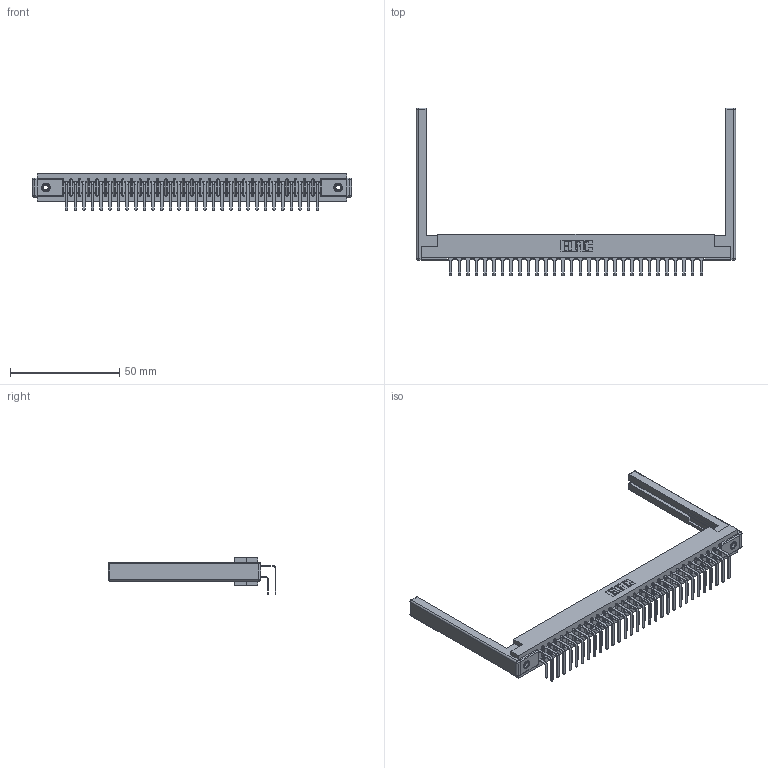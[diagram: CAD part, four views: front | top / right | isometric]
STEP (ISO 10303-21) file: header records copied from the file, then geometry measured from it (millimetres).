
FILE_DESCRIPTION (( 'STEP AP203' ), '1' );
FILE_NAME ('307-030-458-168.STEP', '2020-09-28T11:19:01', ( '' ), ( '' ), 'SwSTEP 2.0', 'SolidWorks 2020', '' );
FILE_SCHEMA (( 'CONFIG_CONTROL_DESIGN' ));
Length unit declared in the file: inch
Products named in the file (6): 307-030-458-168; 307 Part_.156 Dia Mounting Holes; 307-290-001_558 - 2 (Single); 345-250-001_345-250-001-102; 307-220-068; 307-290-001_558 559 - 1 (Single)
Assembly tree (65 placements, depth 2):
  307-030-458-168
    307 Part_.156 Dia Mounting Holes
    307-290-001_558 559 - 1 (Single)  x30
    307-290-001_558 - 2 (Single)  x30
    307-220-068  x2
    345-250-001_345-250-001-102  x2
Bounding box: 146.3 x 76.92 x 16.8 mm (x, y, z)
Volume: 20119.3 mm3; surface area: 24546.5 mm2
Topology: 65 solids, 65 shells, 3303 faces, 9233 edges, 5970 vertices
Faces by surface type: plane 2138, cylinder 1079, sphere 70, cone 12, torus 4
Entity records: 32364 total; most frequent: CARTESIAN_POINT 5277, ORIENTED_EDGE 5220, DIRECTION 5188, EDGE_CURVE 2610, LINE 1994, VECTOR 1994, VERTEX_POINT 1686, AXIS2_PLACEMENT_3D 1597
